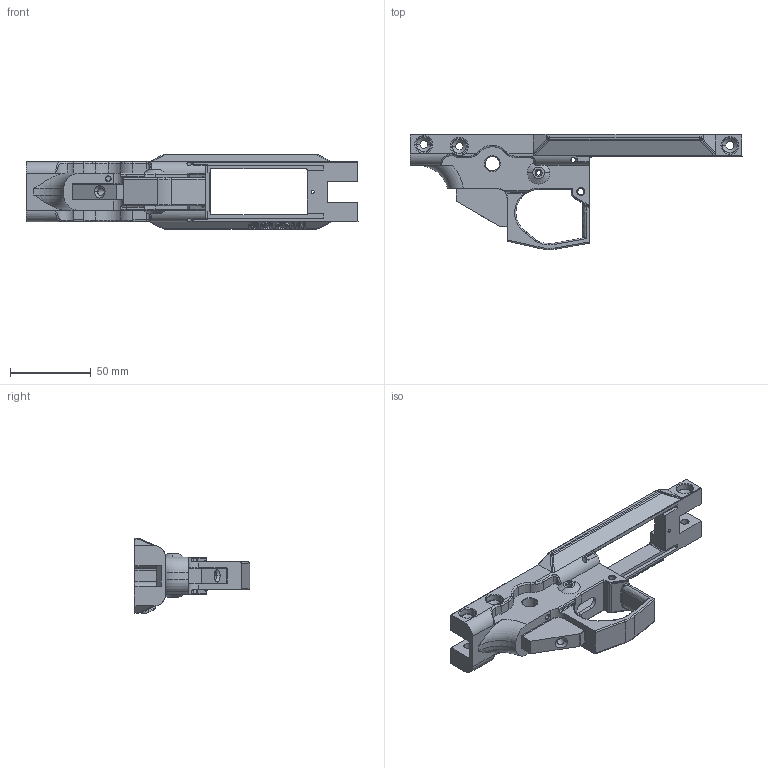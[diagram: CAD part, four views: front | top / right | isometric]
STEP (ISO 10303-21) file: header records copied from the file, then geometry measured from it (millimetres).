
FILE_DESCRIPTION(('STEP AP214'),'1');
FILE_NAME('Mod9 Lower Receiver Final.stp','2020-09-28T22:42:45',(' '),(' '),'Spatial InterOp 3D',' ',' ');
FILE_SCHEMA(('AUTOMOTIVE_DESIGN { 1 0 10303 214 1 1 1 1 }'));
Length unit declared in the file: metre
Products named in the file (1): Body1
Bounding box: 205.1 x 71.28 x 46.33 mm (x, y, z)
Volume: 99554 mm3; surface area: 40040 mm2
Topology: 1 solids, 1 shells, 672 faces, 1813 edges, 1134 vertices
Faces by surface type: cylinder 235, plane 177, bspline 142, cone 61, torus 51, sphere 6
Entity records: 28180 total; most frequent: CARTESIAN_POINT 12023, ORIENTED_EDGE 3602, DIRECTION 3079, EDGE_CURVE 1801, VERTEX_POINT 1134, AXIS2_PLACEMENT_3D 1122, LINE 835, VECTOR 835
